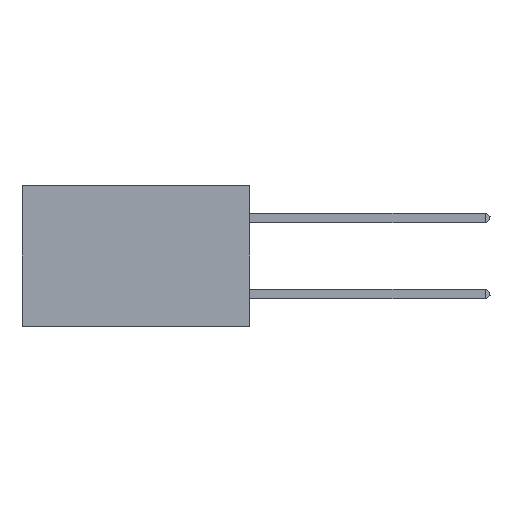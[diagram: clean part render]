
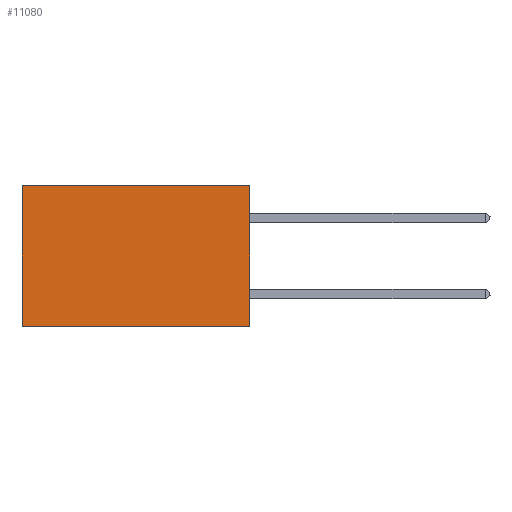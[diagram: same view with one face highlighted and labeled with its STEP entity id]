
A CAD part, left-side view. The second image highlights one B-rep face of the part: STEP entity #11080.
In plain terms, the highlighted planar face has unit normal (-1, 0, 0).
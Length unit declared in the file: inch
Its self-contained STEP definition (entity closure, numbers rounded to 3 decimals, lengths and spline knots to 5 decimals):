
#390 = FACE_OUTER_BOUND ( 'NONE', #9751, .T. ) ;
#2900 = CARTESIAN_POINT ( 'NONE',  ( 0.2875, 0., 0. ) ) ;
#5372 = VERTEX_POINT ( 'NONE', #24050 ) ;
#5442 = CARTESIAN_POINT ( 'NONE',  ( 0.2875, 0., -0.37 ) ) ;
#5536 = AXIS2_PLACEMENT_3D ( 'NONE', #25787, #22498, #8427 ) ;
#8427 = DIRECTION ( 'NONE',  ( 0., 0., -1. ) ) ;
#8727 = PLANE ( 'NONE',  #5536 ) ;
#9751 = EDGE_LOOP ( 'NONE', ( #30799, #25047, #10152, #37714 ) ) ;
#10152 = ORIENTED_EDGE ( 'NONE', *, *, #14968, .F. ) ;
#10845 = VECTOR ( 'NONE', #32947, 39.37008 ) ;
#11080 = ADVANCED_FACE ( 'NONE', ( #390 ), #8727, .F. ) ;
#11670 = CARTESIAN_POINT ( 'NONE',  ( 0.2875, 0.6, 0. ) ) ;
#11869 = DIRECTION ( 'NONE',  ( 0., 0., -1. ) ) ;
#12239 = LINE ( 'NONE', #27317, #14367 ) ;
#12494 = DIRECTION ( 'NONE',  ( 0., 1., 0. ) ) ;
#14367 = VECTOR ( 'NONE', #30825, 39.37008 ) ;
#14968 = EDGE_CURVE ( 'NONE', #34210, #27531, #37784, .T. ) ;
#17119 = VECTOR ( 'NONE', #11869, 39.37008 ) ;
#17988 = VERTEX_POINT ( 'NONE', #11670 ) ;
#18164 = LINE ( 'NONE', #18347, #17119 ) ;
#18347 = CARTESIAN_POINT ( 'NONE',  ( 0.2875, 0.6, 0. ) ) ;
#18989 = EDGE_CURVE ( 'NONE', #17988, #5372, #18164, .T. ) ;
#22498 = DIRECTION ( 'NONE',  ( 1., 0., 0. ) ) ;
#24050 = CARTESIAN_POINT ( 'NONE',  ( 0.2875, 0.6, -0.37 ) ) ;
#25047 = ORIENTED_EDGE ( 'NONE', *, *, #28010, .F. ) ;
#25304 = EDGE_CURVE ( 'NONE', #34210, #17988, #12239, .T. ) ;
#25787 = CARTESIAN_POINT ( 'NONE',  ( 0.2875, 0., 0. ) ) ;
#27317 = CARTESIAN_POINT ( 'NONE',  ( 0.2875, 0., 0. ) ) ;
#27531 = VERTEX_POINT ( 'NONE', #30430 ) ;
#28010 = EDGE_CURVE ( 'NONE', #27531, #5372, #28549, .T. ) ;
#28549 = LINE ( 'NONE', #5442, #34297 ) ;
#30430 = CARTESIAN_POINT ( 'NONE',  ( 0.2875, 0., -0.37 ) ) ;
#30799 = ORIENTED_EDGE ( 'NONE', *, *, #18989, .T. ) ;
#30825 = DIRECTION ( 'NONE',  ( 0., 1., 0. ) ) ;
#32947 = DIRECTION ( 'NONE',  ( 0., 0., -1. ) ) ;
#34210 = VERTEX_POINT ( 'NONE', #2900 ) ;
#34297 = VECTOR ( 'NONE', #12494, 39.37008 ) ;
#37714 = ORIENTED_EDGE ( 'NONE', *, *, #25304, .T. ) ;
#37784 = LINE ( 'NONE', #43737, #10845 ) ;
#43737 = CARTESIAN_POINT ( 'NONE',  ( 0.2875, 0., 0. ) ) ;
